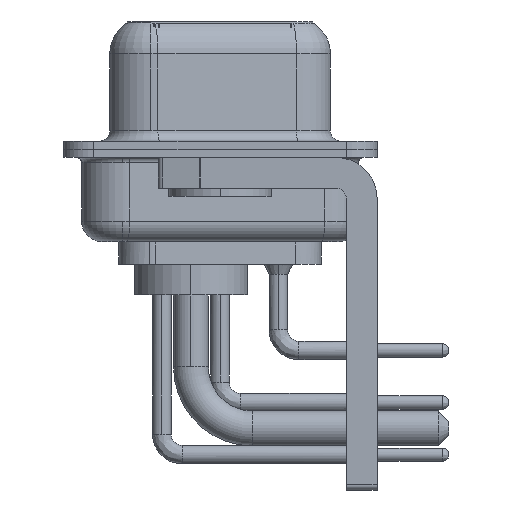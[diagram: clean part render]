
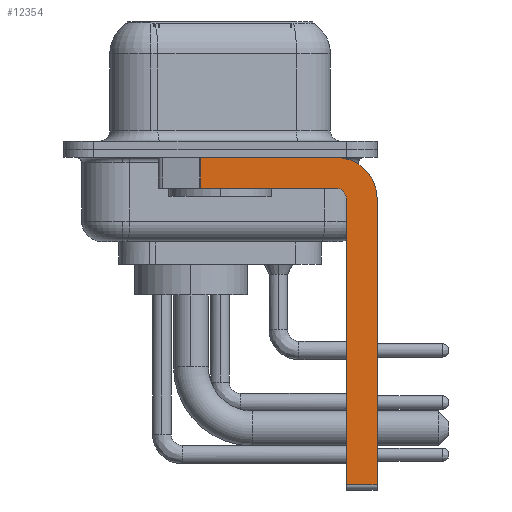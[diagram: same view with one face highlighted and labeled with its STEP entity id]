
A CAD part, left-side view. The second image highlights one B-rep face of the part: STEP entity #12354.
In plain terms, the highlighted planar face has unit normal (-1, 0, 0).
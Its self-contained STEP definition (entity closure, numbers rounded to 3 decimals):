
#96 = CARTESIAN_POINT ( 'NONE',  ( -2.9, -5.65, -2.4 ) ) ;
#697 = VECTOR ( 'NONE', #24460, 1000. ) ;
#2164 = CARTESIAN_POINT ( 'NONE',  ( -2.9, -7.65, -2.4 ) ) ;
#2899 = DIRECTION ( 'NONE',  ( 0., 0., -1. ) ) ;
#3083 = EDGE_CURVE ( 'NONE', #26490, #28251, #19842, .T. ) ;
#3398 = CARTESIAN_POINT ( 'NONE',  ( -2.9, -6.15, -16.35 ) ) ;
#3521 = LINE ( 'NONE', #29863, #23070 ) ;
#6520 = CARTESIAN_POINT ( 'NONE',  ( -2.9, -5.65, -1.9 ) ) ;
#6598 = EDGE_LOOP ( 'NONE', ( #8293, #12613, #17420, #19647, #20073, #10056, #24953, #19211 ) ) ;
#7239 = VERTEX_POINT ( 'NONE', #6520 ) ;
#8038 = CIRCLE ( 'NONE', #27646, 2. ) ;
#8293 = ORIENTED_EDGE ( 'NONE', *, *, #29436, .F. ) ;
#9335 = CARTESIAN_POINT ( 'NONE',  ( -2.9, -5.65, -16.35 ) ) ;
#10056 = ORIENTED_EDGE ( 'NONE', *, *, #3083, .T. ) ;
#11135 = CARTESIAN_POINT ( 'NONE',  ( -2.9, 3., -0.4 ) ) ;
#12347 = VECTOR ( 'NONE', #24504, 1000. ) ;
#12354 = ADVANCED_FACE ( 'NONE', ( #18401 ), #24013, .F. ) ;
#12397 = CIRCLE ( 'NONE', #24149, 0.5 ) ;
#12613 = ORIENTED_EDGE ( 'NONE', *, *, #18473, .T. ) ;
#12760 = VERTEX_POINT ( 'NONE', #24668 ) ;
#13688 = DIRECTION ( 'NONE',  ( 1., 0., 0. ) ) ;
#13863 = CARTESIAN_POINT ( 'NONE',  ( -2.9, -5.65, -2.4 ) ) ;
#14243 = DIRECTION ( 'NONE',  ( 0., 0., -1. ) ) ;
#14712 = LINE ( 'NONE', #28569, #18462 ) ;
#14720 = VERTEX_POINT ( 'NONE', #14807 ) ;
#14807 = CARTESIAN_POINT ( 'NONE',  ( -2.9, 0.978, -1.9 ) ) ;
#15533 = DIRECTION ( 'NONE',  ( 0., 1., 0. ) ) ;
#16139 = EDGE_CURVE ( 'NONE', #32322, #28251, #3521, .T. ) ;
#17420 = ORIENTED_EDGE ( 'NONE', *, *, #18707, .F. ) ;
#17890 = CARTESIAN_POINT ( 'NONE',  ( -2.9, -6.15, -2.4 ) ) ;
#18009 = CARTESIAN_POINT ( 'NONE',  ( -2.9, -5.65, -0.4 ) ) ;
#18209 = EDGE_CURVE ( 'NONE', #26490, #19963, #14712, .T. ) ;
#18401 = FACE_OUTER_BOUND ( 'NONE', #6598, .T. ) ;
#18462 = VECTOR ( 'NONE', #31045, 1000. ) ;
#18473 = EDGE_CURVE ( 'NONE', #12760, #14720, #30132, .T. ) ;
#18613 = VECTOR ( 'NONE', #28456, 1000. ) ;
#18707 = EDGE_CURVE ( 'NONE', #7239, #14720, #26892, .T. ) ;
#19211 = ORIENTED_EDGE ( 'NONE', *, *, #21549, .F. ) ;
#19308 = EDGE_CURVE ( 'NONE', #19963, #7239, #12397, .T. ) ;
#19647 = ORIENTED_EDGE ( 'NONE', *, *, #19308, .F. ) ;
#19842 = LINE ( 'NONE', #9335, #18613 ) ;
#19963 = VERTEX_POINT ( 'NONE', #17890 ) ;
#20073 = ORIENTED_EDGE ( 'NONE', *, *, #18209, .F. ) ;
#20685 = DIRECTION ( 'NONE',  ( 0., 0., -1. ) ) ;
#21503 = DIRECTION ( 'NONE',  ( 1., 0., 0. ) ) ;
#21549 = EDGE_CURVE ( 'NONE', #28931, #32322, #8038, .T. ) ;
#22034 = CARTESIAN_POINT ( 'NONE',  ( -2.9, 0.978, -1.9 ) ) ;
#23070 = VECTOR ( 'NONE', #14243, 1000. ) ;
#23374 = AXIS2_PLACEMENT_3D ( 'NONE', #34237, #13688, #20685 ) ;
#24013 = PLANE ( 'NONE',  #23374 ) ;
#24149 = AXIS2_PLACEMENT_3D ( 'NONE', #13863, #31797, #26507 ) ;
#24460 = DIRECTION ( 'NONE',  ( 0., -1., 0. ) ) ;
#24504 = DIRECTION ( 'NONE',  ( 0., 0., -1. ) ) ;
#24668 = CARTESIAN_POINT ( 'NONE',  ( -2.9, 0.978, -0.4 ) ) ;
#24953 = ORIENTED_EDGE ( 'NONE', *, *, #16139, .F. ) ;
#25305 = CARTESIAN_POINT ( 'NONE',  ( -2.9, -7.65, -16.35 ) ) ;
#26490 = VERTEX_POINT ( 'NONE', #3398 ) ;
#26507 = DIRECTION ( 'NONE',  ( 0., 0., 1. ) ) ;
#26892 = LINE ( 'NONE', #31528, #29168 ) ;
#27646 = AXIS2_PLACEMENT_3D ( 'NONE', #96, #21503, #2899 ) ;
#28251 = VERTEX_POINT ( 'NONE', #25305 ) ;
#28456 = DIRECTION ( 'NONE',  ( 0., -1., 0. ) ) ;
#28569 = CARTESIAN_POINT ( 'NONE',  ( -2.9, -6.15, -16.6 ) ) ;
#28931 = VERTEX_POINT ( 'NONE', #18009 ) ;
#29168 = VECTOR ( 'NONE', #15533, 1000. ) ;
#29436 = EDGE_CURVE ( 'NONE', #12760, #28931, #32042, .T. ) ;
#29863 = CARTESIAN_POINT ( 'NONE',  ( -2.9, -7.65, -2.4 ) ) ;
#30132 = LINE ( 'NONE', #22034, #12347 ) ;
#31045 = DIRECTION ( 'NONE',  ( 0., 0., 1. ) ) ;
#31528 = CARTESIAN_POINT ( 'NONE',  ( -2.9, -5.65, -1.9 ) ) ;
#31797 = DIRECTION ( 'NONE',  ( -1., 0., 0. ) ) ;
#32042 = LINE ( 'NONE', #11135, #697 ) ;
#32322 = VERTEX_POINT ( 'NONE', #2164 ) ;
#34237 = CARTESIAN_POINT ( 'NONE',  ( -2.9, -5.65, -2.4 ) ) ;
